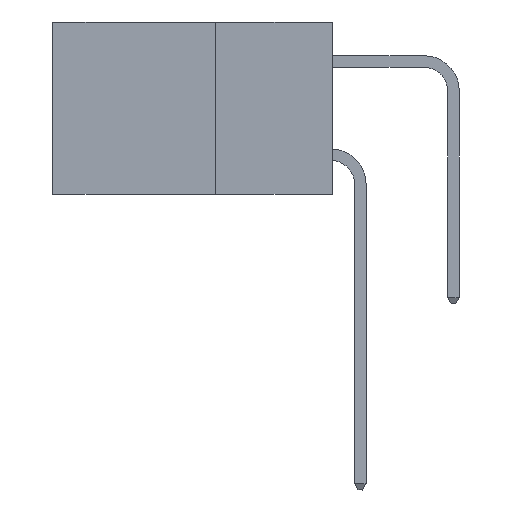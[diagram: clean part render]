
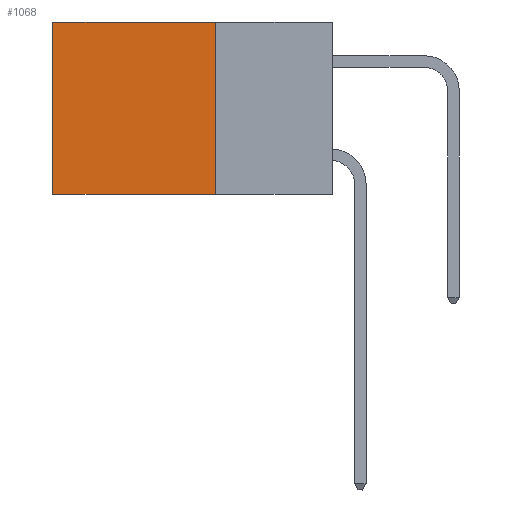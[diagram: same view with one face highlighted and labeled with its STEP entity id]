
A CAD part, left-side view. The second image highlights one B-rep face of the part: STEP entity #1068.
In plain terms, the highlighted planar face has unit normal (-1, 0, 0).
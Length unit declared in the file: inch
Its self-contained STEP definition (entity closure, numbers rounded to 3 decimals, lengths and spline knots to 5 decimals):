
#1068 = ADVANCED_FACE ( 'NONE', ( #10360 ), #9427, .F. ) ;
#1711 = LINE ( 'NONE', #9003, #2514 ) ;
#2455 = VERTEX_POINT ( 'NONE', #3346 ) ;
#2514 = VECTOR ( 'NONE', #10207, 39.37008 ) ;
#2890 = LINE ( 'NONE', #12214, #8630 ) ;
#2989 = VECTOR ( 'NONE', #6817, 39.37008 ) ;
#3346 = CARTESIAN_POINT ( 'NONE',  ( 0.298, 0.25, 0. ) ) ;
#3954 = CARTESIAN_POINT ( 'NONE',  ( 0.298, 0.25, 0. ) ) ;
#4197 = VERTEX_POINT ( 'NONE', #9679 ) ;
#5003 = DIRECTION ( 'NONE',  ( 0., 0., -1. ) ) ;
#6024 = VERTEX_POINT ( 'NONE', #11234 ) ;
#6817 = DIRECTION ( 'NONE',  ( 0., 1., 0. ) ) ;
#7495 = EDGE_CURVE ( 'NONE', #6024, #4197, #10246, .T. ) ;
#7626 = AXIS2_PLACEMENT_3D ( 'NONE', #3954, #11352, #5003 ) ;
#8062 = LINE ( 'NONE', #13476, #10524 ) ;
#8504 = EDGE_CURVE ( 'NONE', #8575, #4197, #8062, .T. ) ;
#8575 = VERTEX_POINT ( 'NONE', #12738 ) ;
#8630 = VECTOR ( 'NONE', #8963, 39.37008 ) ;
#8963 = DIRECTION ( 'NONE',  ( 0., 0., -1. ) ) ;
#9003 = CARTESIAN_POINT ( 'NONE',  ( 0.298, 0.25, 0. ) ) ;
#9427 = PLANE ( 'NONE',  #7626 ) ;
#9676 = ORIENTED_EDGE ( 'NONE', *, *, #10947, .F. ) ;
#9679 = CARTESIAN_POINT ( 'NONE',  ( 0.298, 0.6, -0.37 ) ) ;
#9722 = ORIENTED_EDGE ( 'NONE', *, *, #12380, .T. ) ;
#10207 = DIRECTION ( 'NONE',  ( 0., 1., 0. ) ) ;
#10246 = LINE ( 'NONE', #12094, #2989 ) ;
#10313 = DIRECTION ( 'NONE',  ( 0., 0., -1. ) ) ;
#10360 = FACE_OUTER_BOUND ( 'NONE', #11065, .T. ) ;
#10524 = VECTOR ( 'NONE', #10313, 39.37008 ) ;
#10835 = ORIENTED_EDGE ( 'NONE', *, *, #7495, .F. ) ;
#10947 = EDGE_CURVE ( 'NONE', #2455, #6024, #2890, .T. ) ;
#11065 = EDGE_LOOP ( 'NONE', ( #12537, #10835, #9676, #9722 ) ) ;
#11234 = CARTESIAN_POINT ( 'NONE',  ( 0.298, 0.25, -0.37 ) ) ;
#11352 = DIRECTION ( 'NONE',  ( 1., 0., 0. ) ) ;
#12094 = CARTESIAN_POINT ( 'NONE',  ( 0.298, 0.25, -0.37 ) ) ;
#12214 = CARTESIAN_POINT ( 'NONE',  ( 0.298, 0.25, 0. ) ) ;
#12380 = EDGE_CURVE ( 'NONE', #2455, #8575, #1711, .T. ) ;
#12537 = ORIENTED_EDGE ( 'NONE', *, *, #8504, .T. ) ;
#12738 = CARTESIAN_POINT ( 'NONE',  ( 0.298, 0.6, 0. ) ) ;
#13476 = CARTESIAN_POINT ( 'NONE',  ( 0.298, 0.6, 0. ) ) ;
